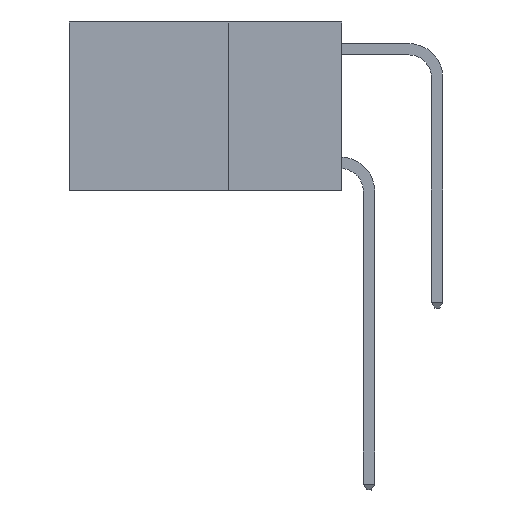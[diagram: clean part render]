
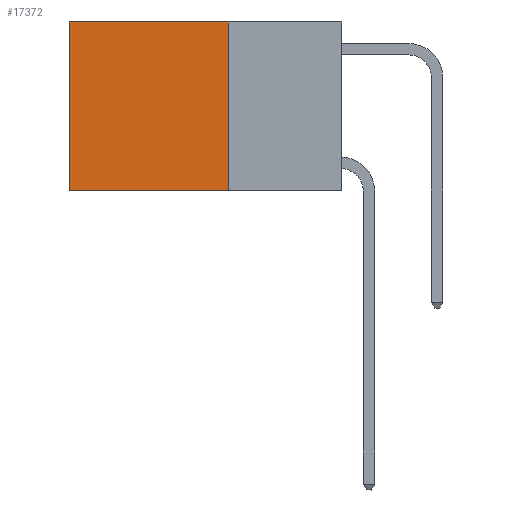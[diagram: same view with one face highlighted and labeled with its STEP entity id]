
A CAD part, left-side view. The second image highlights one B-rep face of the part: STEP entity #17372.
In plain terms, the highlighted planar face has unit normal (-1, 0, 0).
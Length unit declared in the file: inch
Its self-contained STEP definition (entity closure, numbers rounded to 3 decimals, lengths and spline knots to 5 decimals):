
#583 = CARTESIAN_POINT ( 'NONE',  ( 0.2625, 0.25, -0.37 ) ) ;
#662 = DIRECTION ( 'NONE',  ( 0., 0., -1. ) ) ;
#720 = AXIS2_PLACEMENT_3D ( 'NONE', #2675, #5617, #15589 ) ;
#1068 = ORIENTED_EDGE ( 'NONE', *, *, #13597, .T. ) ;
#1399 = LINE ( 'NONE', #1540, #14824 ) ;
#1536 = CARTESIAN_POINT ( 'NONE',  ( 0.2625, 0.25, -0.37 ) ) ;
#1540 = CARTESIAN_POINT ( 'NONE',  ( 0.2625, 0.25, 0. ) ) ;
#2388 = DIRECTION ( 'NONE',  ( 0., 1., 0. ) ) ;
#2675 = CARTESIAN_POINT ( 'NONE',  ( 0.2625, 0.25, 0. ) ) ;
#2738 = CARTESIAN_POINT ( 'NONE',  ( 0.2625, 0.25, 0. ) ) ;
#2791 = ORIENTED_EDGE ( 'NONE', *, *, #4003, .T. ) ;
#2876 = ORIENTED_EDGE ( 'NONE', *, *, #11851, .F. ) ;
#3277 = VERTEX_POINT ( 'NONE', #2738 ) ;
#3413 = CARTESIAN_POINT ( 'NONE',  ( 0.2625, 0.6, -0.37 ) ) ;
#4003 = EDGE_CURVE ( 'NONE', #12359, #13396, #14541, .T. ) ;
#5617 = DIRECTION ( 'NONE',  ( 1., 0., 0. ) ) ;
#5620 = VECTOR ( 'NONE', #2388, 39.37008 ) ;
#6014 = VERTEX_POINT ( 'NONE', #583 ) ;
#7411 = VECTOR ( 'NONE', #662, 39.37008 ) ;
#8380 = PLANE ( 'NONE',  #720 ) ;
#8606 = ORIENTED_EDGE ( 'NONE', *, *, #9936, .F. ) ;
#9127 = LINE ( 'NONE', #1536, #15784 ) ;
#9319 = CARTESIAN_POINT ( 'NONE',  ( 0.2625, 0.6, 0. ) ) ;
#9718 = FACE_OUTER_BOUND ( 'NONE', #13610, .T. ) ;
#9936 = EDGE_CURVE ( 'NONE', #6014, #13396, #9127, .T. ) ;
#11851 = EDGE_CURVE ( 'NONE', #3277, #6014, #1399, .T. ) ;
#12359 = VERTEX_POINT ( 'NONE', #15478 ) ;
#13053 = DIRECTION ( 'NONE',  ( 0., 1., 0. ) ) ;
#13239 = LINE ( 'NONE', #15233, #5620 ) ;
#13396 = VERTEX_POINT ( 'NONE', #3413 ) ;
#13597 = EDGE_CURVE ( 'NONE', #3277, #12359, #13239, .T. ) ;
#13610 = EDGE_LOOP ( 'NONE', ( #2791, #8606, #2876, #1068 ) ) ;
#14541 = LINE ( 'NONE', #9319, #7411 ) ;
#14824 = VECTOR ( 'NONE', #15857, 39.37008 ) ;
#15233 = CARTESIAN_POINT ( 'NONE',  ( 0.2625, 0.25, 0. ) ) ;
#15478 = CARTESIAN_POINT ( 'NONE',  ( 0.2625, 0.6, 0. ) ) ;
#15589 = DIRECTION ( 'NONE',  ( 0., 0., -1. ) ) ;
#15784 = VECTOR ( 'NONE', #13053, 39.37008 ) ;
#15857 = DIRECTION ( 'NONE',  ( 0., 0., -1. ) ) ;
#17372 = ADVANCED_FACE ( 'NONE', ( #9718 ), #8380, .F. ) ;
